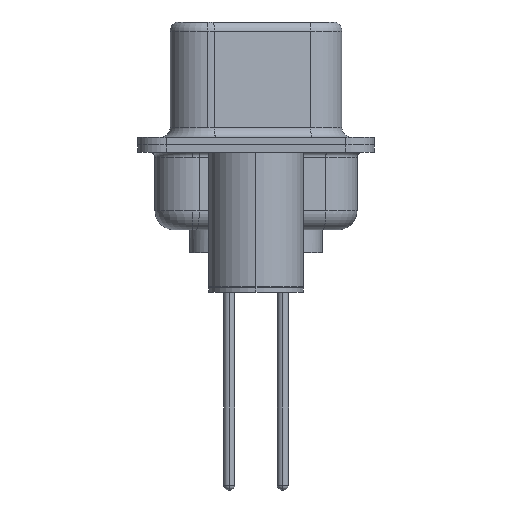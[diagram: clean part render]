
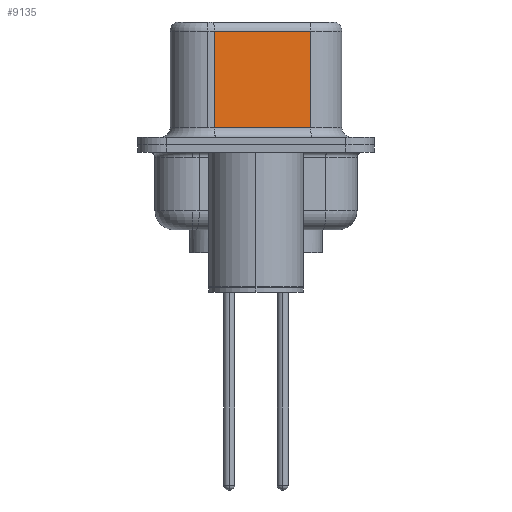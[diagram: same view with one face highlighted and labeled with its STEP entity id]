
A CAD part, left-side view. The second image highlights one B-rep face of the part: STEP entity #9135.
In plain terms, the highlighted planar face has unit normal (-0.985, -0.174, 0).
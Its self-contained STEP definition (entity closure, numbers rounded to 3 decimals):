
#90 = DIRECTION ( 'NONE',  ( 0., 0., -1. ) ) ;
#386 = DIRECTION ( 'NONE',  ( -0.174, 0.985, 0. ) ) ;
#448 = ORIENTED_EDGE ( 'NONE', *, *, #12410, .F. ) ;
#664 = CARTESIAN_POINT ( 'NONE',  ( 4.555, -2.897, 0.9 ) ) ;
#790 = DIRECTION ( 'NONE',  ( 0., 0., -1. ) ) ;
#954 = LINE ( 'NONE', #10431, #8625 ) ;
#1231 = CARTESIAN_POINT ( 'NONE',  ( 4.555, -2.897, 0.9 ) ) ;
#2196 = EDGE_LOOP ( 'NONE', ( #448, #3517, #11668, #11041 ) ) ;
#3157 = EDGE_CURVE ( 'NONE', #12310, #8455, #12543, .T. ) ;
#3517 = ORIENTED_EDGE ( 'NONE', *, *, #3157, .T. ) ;
#3621 = FACE_OUTER_BOUND ( 'NONE', #2196, .T. ) ;
#3984 = LINE ( 'NONE', #9477, #14208 ) ;
#4604 = CARTESIAN_POINT ( 'NONE',  ( 4.555, -2.897, 6.02 ) ) ;
#5603 = CARTESIAN_POINT ( 'NONE',  ( 3.655, 2.203, 0.9 ) ) ;
#7398 = EDGE_CURVE ( 'NONE', #8455, #13082, #3984, .T. ) ;
#7705 = PLANE ( 'NONE',  #10025 ) ;
#8455 = VERTEX_POINT ( 'NONE', #14207 ) ;
#8623 = CARTESIAN_POINT ( 'NONE',  ( 4.555, -2.897, 6.02 ) ) ;
#8625 = VECTOR ( 'NONE', #790, 1000. ) ;
#9135 = ADVANCED_FACE ( 'NONE', ( #3621 ), #7705, .F. ) ;
#9191 = DIRECTION ( 'NONE',  ( -0.174, 0.985, 0. ) ) ;
#9477 = CARTESIAN_POINT ( 'NONE',  ( 3.655, 2.203, 6.52 ) ) ;
#10025 = AXIS2_PLACEMENT_3D ( 'NONE', #10258, #11761, #9191 ) ;
#10258 = CARTESIAN_POINT ( 'NONE',  ( 4.555, -2.897, 6.52 ) ) ;
#10431 = CARTESIAN_POINT ( 'NONE',  ( 4.555, -2.897, 6.52 ) ) ;
#10460 = DIRECTION ( 'NONE',  ( 0.174, -0.985, 0. ) ) ;
#11041 = ORIENTED_EDGE ( 'NONE', *, *, #14779, .T. ) ;
#11668 = ORIENTED_EDGE ( 'NONE', *, *, #7398, .T. ) ;
#11761 = DIRECTION ( 'NONE',  ( 0.985, 0.174, 0. ) ) ;
#12310 = VERTEX_POINT ( 'NONE', #4604 ) ;
#12410 = EDGE_CURVE ( 'NONE', #12310, #17478, #954, .T. ) ;
#12543 = LINE ( 'NONE', #8623, #14404 ) ;
#12631 = VECTOR ( 'NONE', #10460, 1000. ) ;
#13082 = VERTEX_POINT ( 'NONE', #5603 ) ;
#14144 = LINE ( 'NONE', #664, #12631 ) ;
#14207 = CARTESIAN_POINT ( 'NONE',  ( 3.655, 2.203, 6.02 ) ) ;
#14208 = VECTOR ( 'NONE', #90, 1000. ) ;
#14404 = VECTOR ( 'NONE', #386, 1000. ) ;
#14779 = EDGE_CURVE ( 'NONE', #13082, #17478, #14144, .T. ) ;
#17478 = VERTEX_POINT ( 'NONE', #1231 ) ;
